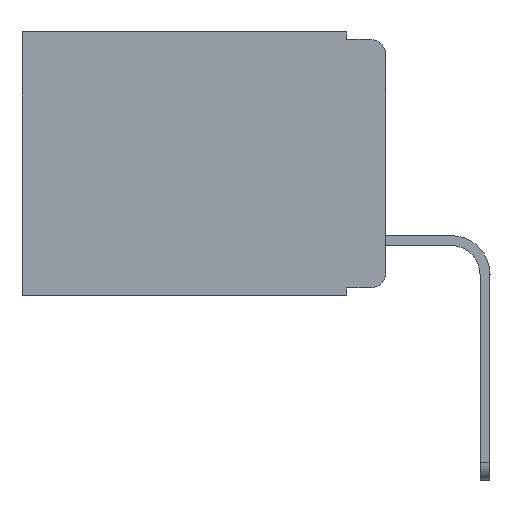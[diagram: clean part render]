
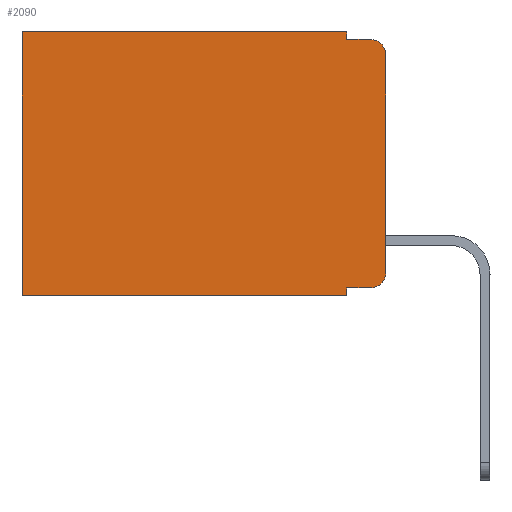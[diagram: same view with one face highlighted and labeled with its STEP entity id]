
A CAD part, left-side view. The second image highlights one B-rep face of the part: STEP entity #2090.
In plain terms, the highlighted planar face has unit normal (-1, 0, 0).
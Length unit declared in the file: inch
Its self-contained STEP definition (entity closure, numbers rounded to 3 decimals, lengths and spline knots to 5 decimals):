
#35 = ORIENTED_EDGE ( 'NONE', *, *, #14051, .F. ) ;
#439 = AXIS2_PLACEMENT_3D ( 'NONE', #19161, #12662, #15761 ) ;
#855 = VERTEX_POINT ( 'NONE', #9753 ) ;
#1564 = ORIENTED_EDGE ( 'NONE', *, *, #4474, .F. ) ;
#2086 = LINE ( 'NONE', #20257, #14112 ) ;
#2090 = ADVANCED_FACE ( 'NONE', ( #6135 ), #9674, .F. ) ;
#2860 = VERTEX_POINT ( 'NONE', #16067 ) ;
#3227 = VERTEX_POINT ( 'NONE', #20062 ) ;
#3407 = ORIENTED_EDGE ( 'NONE', *, *, #8060, .F. ) ;
#3954 = EDGE_CURVE ( 'NONE', #10470, #2860, #11680, .T. ) ;
#4273 = DIRECTION ( 'NONE',  ( -1., 0., 0. ) ) ;
#4275 = VERTEX_POINT ( 'NONE', #9690 ) ;
#4310 = CARTESIAN_POINT ( 'NONE',  ( 0.298, 0., 0. ) ) ;
#4474 = EDGE_CURVE ( 'NONE', #15921, #4275, #2086, .T. ) ;
#4947 = DIRECTION ( 'NONE',  ( 0., 0., -1. ) ) ;
#5775 = DIRECTION ( 'NONE',  ( 0., -1., 0. ) ) ;
#6135 = FACE_OUTER_BOUND ( 'NONE', #20961, .T. ) ;
#6258 = VECTOR ( 'NONE', #13338, 39.37008 ) ;
#6430 = EDGE_CURVE ( 'NONE', #11011, #20208, #11956, .T. ) ;
#6503 = CARTESIAN_POINT ( 'NONE',  ( 0.298, 0.051, -0.01 ) ) ;
#6943 = CARTESIAN_POINT ( 'NONE',  ( 0.298, 0.051, 0. ) ) ;
#7455 = EDGE_CURVE ( 'NONE', #19222, #855, #13984, .T. ) ;
#7552 = DIRECTION ( 'NONE',  ( 0., 0., -1. ) ) ;
#7913 = CARTESIAN_POINT ( 'NONE',  ( 0.298, 0., 0. ) ) ;
#8060 = EDGE_CURVE ( 'NONE', #11011, #13120, #15237, .T. ) ;
#8658 = EDGE_CURVE ( 'NONE', #3227, #19222, #20032, .T. ) ;
#9062 = CARTESIAN_POINT ( 'NONE',  ( 0.298, 0.02, -0.333 ) ) ;
#9361 = VECTOR ( 'NONE', #15075, 39.37008 ) ;
#9456 = DIRECTION ( 'NONE',  ( 1., 0., 0. ) ) ;
#9674 = PLANE ( 'NONE',  #20721 ) ;
#9690 = CARTESIAN_POINT ( 'NONE',  ( 0.298, 0.473, -0.343 ) ) ;
#9753 = CARTESIAN_POINT ( 'NONE',  ( 0.298, 0., -0.313 ) ) ;
#9905 = VECTOR ( 'NONE', #20992, 39.37008 ) ;
#10190 = LINE ( 'NONE', #4310, #17336 ) ;
#10302 = CARTESIAN_POINT ( 'NONE',  ( 0.298, 0.473, 0. ) ) ;
#10436 = LINE ( 'NONE', #15778, #19335 ) ;
#10470 = VERTEX_POINT ( 'NONE', #18280 ) ;
#11011 = VERTEX_POINT ( 'NONE', #6943 ) ;
#11680 = CIRCLE ( 'NONE', #14912, 0.02 ) ;
#11956 = LINE ( 'NONE', #16222, #9905 ) ;
#12477 = CARTESIAN_POINT ( 'NONE',  ( 0.298, 0.02, -0.03 ) ) ;
#12542 = DIRECTION ( 'NONE',  ( 0., 0., -1. ) ) ;
#12662 = DIRECTION ( 'NONE',  ( -1., 0., 0. ) ) ;
#13120 = VERTEX_POINT ( 'NONE', #6503 ) ;
#13338 = DIRECTION ( 'NONE',  ( 0., -1., 0. ) ) ;
#13931 = ORIENTED_EDGE ( 'NONE', *, *, #3954, .T. ) ;
#13984 = CIRCLE ( 'NONE', #439, 0.02 ) ;
#14032 = CARTESIAN_POINT ( 'NONE',  ( 0.298, 0.051, 0. ) ) ;
#14051 = EDGE_CURVE ( 'NONE', #13120, #2860, #19640, .T. ) ;
#14112 = VECTOR ( 'NONE', #16897, 39.37008 ) ;
#14193 = EDGE_CURVE ( 'NONE', #10470, #855, #10190, .T. ) ;
#14774 = EDGE_CURVE ( 'NONE', #3227, #15921, #10436, .T. ) ;
#14912 = AXIS2_PLACEMENT_3D ( 'NONE', #12477, #4273, #12542 ) ;
#14929 = CARTESIAN_POINT ( 'NONE',  ( 0.298, 0.473, 0. ) ) ;
#14957 = ORIENTED_EDGE ( 'NONE', *, *, #14774, .F. ) ;
#15075 = DIRECTION ( 'NONE',  ( 0., 0., -1. ) ) ;
#15237 = LINE ( 'NONE', #14032, #20808 ) ;
#15238 = ORIENTED_EDGE ( 'NONE', *, *, #21129, .T. ) ;
#15314 = ORIENTED_EDGE ( 'NONE', *, *, #7455, .T. ) ;
#15398 = CARTESIAN_POINT ( 'NONE',  ( 0.298, 0.051, -0.01 ) ) ;
#15678 = DIRECTION ( 'NONE',  ( 0., 0., -1. ) ) ;
#15761 = DIRECTION ( 'NONE',  ( 0., 0., -1. ) ) ;
#15778 = CARTESIAN_POINT ( 'NONE',  ( 0.298, 0.051, 0. ) ) ;
#15921 = VERTEX_POINT ( 'NONE', #21074 ) ;
#16050 = ORIENTED_EDGE ( 'NONE', *, *, #8658, .T. ) ;
#16067 = CARTESIAN_POINT ( 'NONE',  ( 0.298, 0.02, -0.01 ) ) ;
#16222 = CARTESIAN_POINT ( 'NONE',  ( 0.298, 0., 0. ) ) ;
#16328 = VECTOR ( 'NONE', #5775, 39.37008 ) ;
#16418 = CARTESIAN_POINT ( 'NONE',  ( 0.298, 0.051, -0.333 ) ) ;
#16897 = DIRECTION ( 'NONE',  ( 0., 1., 0. ) ) ;
#17171 = ORIENTED_EDGE ( 'NONE', *, *, #6430, .T. ) ;
#17336 = VECTOR ( 'NONE', #7552, 39.37008 ) ;
#17484 = DIRECTION ( 'NONE',  ( 0., 0., -1. ) ) ;
#17519 = LINE ( 'NONE', #14929, #9361 ) ;
#18280 = CARTESIAN_POINT ( 'NONE',  ( 0.298, 0., -0.03 ) ) ;
#19161 = CARTESIAN_POINT ( 'NONE',  ( 0.298, 0.02, -0.313 ) ) ;
#19222 = VERTEX_POINT ( 'NONE', #9062 ) ;
#19335 = VECTOR ( 'NONE', #17484, 39.37008 ) ;
#19640 = LINE ( 'NONE', #15398, #16328 ) ;
#20032 = LINE ( 'NONE', #16418, #6258 ) ;
#20062 = CARTESIAN_POINT ( 'NONE',  ( 0.298, 0.051, -0.333 ) ) ;
#20145 = ORIENTED_EDGE ( 'NONE', *, *, #14193, .F. ) ;
#20208 = VERTEX_POINT ( 'NONE', #10302 ) ;
#20257 = CARTESIAN_POINT ( 'NONE',  ( 0.298, 0., -0.343 ) ) ;
#20721 = AXIS2_PLACEMENT_3D ( 'NONE', #7913, #9456, #4947 ) ;
#20808 = VECTOR ( 'NONE', #15678, 39.37008 ) ;
#20961 = EDGE_LOOP ( 'NONE', ( #20145, #13931, #35, #3407, #17171, #15238, #1564, #14957, #16050, #15314 ) ) ;
#20992 = DIRECTION ( 'NONE',  ( 0., 1., 0. ) ) ;
#21074 = CARTESIAN_POINT ( 'NONE',  ( 0.298, 0.051, -0.343 ) ) ;
#21129 = EDGE_CURVE ( 'NONE', #20208, #4275, #17519, .T. ) ;
